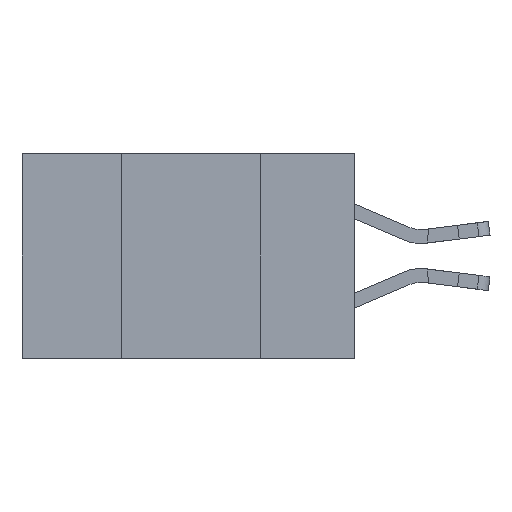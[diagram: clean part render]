
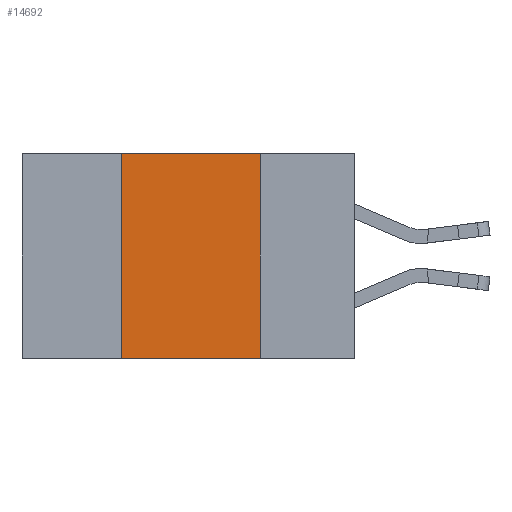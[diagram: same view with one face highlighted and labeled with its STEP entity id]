
A CAD part, left-side view. The second image highlights one B-rep face of the part: STEP entity #14692.
In plain terms, the highlighted planar face has unit normal (-1, 0, 0).
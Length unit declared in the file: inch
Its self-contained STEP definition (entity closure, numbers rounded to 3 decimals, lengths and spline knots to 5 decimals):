
#297 = DIRECTION ( 'NONE',  ( 0., 0., -1. ) ) ;
#569 = VERTEX_POINT ( 'NONE', #2504 ) ;
#1338 = CARTESIAN_POINT ( 'NONE',  ( 0., 0.6, -0.37 ) ) ;
#2504 = CARTESIAN_POINT ( 'NONE',  ( 0., 0.17, -0.37 ) ) ;
#2977 = CARTESIAN_POINT ( 'NONE',  ( 0., 0.42, -0.37 ) ) ;
#4148 = LINE ( 'NONE', #16733, #14920 ) ;
#5306 = EDGE_CURVE ( 'NONE', #13377, #9232, #5908, .T. ) ;
#5689 = EDGE_CURVE ( 'NONE', #9232, #9872, #7166, .T. ) ;
#5908 = LINE ( 'NONE', #12750, #12729 ) ;
#7007 = PLANE ( 'NONE',  #8415 ) ;
#7166 = LINE ( 'NONE', #8077, #9934 ) ;
#7620 = EDGE_CURVE ( 'NONE', #9872, #569, #4148, .T. ) ;
#7667 = EDGE_LOOP ( 'NONE', ( #16644, #11616, #12060, #16438 ) ) ;
#8077 = CARTESIAN_POINT ( 'NONE',  ( 0., 0.6, 0. ) ) ;
#8382 = DIRECTION ( 'NONE',  ( 1., 0., 0. ) ) ;
#8415 = AXIS2_PLACEMENT_3D ( 'NONE', #16446, #8382, #297 ) ;
#8687 = DIRECTION ( 'NONE',  ( 0., 0., 1. ) ) ;
#9232 = VERTEX_POINT ( 'NONE', #14782 ) ;
#9366 = CARTESIAN_POINT ( 'NONE',  ( 0., 0.17, 0. ) ) ;
#9872 = VERTEX_POINT ( 'NONE', #9366 ) ;
#9934 = VECTOR ( 'NONE', #13562, 39.37008 ) ;
#11616 = ORIENTED_EDGE ( 'NONE', *, *, #5689, .F. ) ;
#12060 = ORIENTED_EDGE ( 'NONE', *, *, #5306, .F. ) ;
#12729 = VECTOR ( 'NONE', #8687, 39.37008 ) ;
#12750 = CARTESIAN_POINT ( 'NONE',  ( 0., 0.42, 0. ) ) ;
#13377 = VERTEX_POINT ( 'NONE', #2977 ) ;
#13547 = DIRECTION ( 'NONE',  ( 0., -1., 0. ) ) ;
#13562 = DIRECTION ( 'NONE',  ( 0., -1., 0. ) ) ;
#13941 = VECTOR ( 'NONE', #13547, 39.37008 ) ;
#14692 = ADVANCED_FACE ( 'NONE', ( #15208 ), #7007, .F. ) ;
#14782 = CARTESIAN_POINT ( 'NONE',  ( 0., 0.42, 0. ) ) ;
#14920 = VECTOR ( 'NONE', #15402, 39.37008 ) ;
#15134 = LINE ( 'NONE', #1338, #13941 ) ;
#15208 = FACE_OUTER_BOUND ( 'NONE', #7667, .T. ) ;
#15216 = EDGE_CURVE ( 'NONE', #13377, #569, #15134, .T. ) ;
#15402 = DIRECTION ( 'NONE',  ( 0., 0., -1. ) ) ;
#16438 = ORIENTED_EDGE ( 'NONE', *, *, #15216, .T. ) ;
#16446 = CARTESIAN_POINT ( 'NONE',  ( 0., 0.6, 0. ) ) ;
#16644 = ORIENTED_EDGE ( 'NONE', *, *, #7620, .F. ) ;
#16733 = CARTESIAN_POINT ( 'NONE',  ( 0., 0.17, 0. ) ) ;
